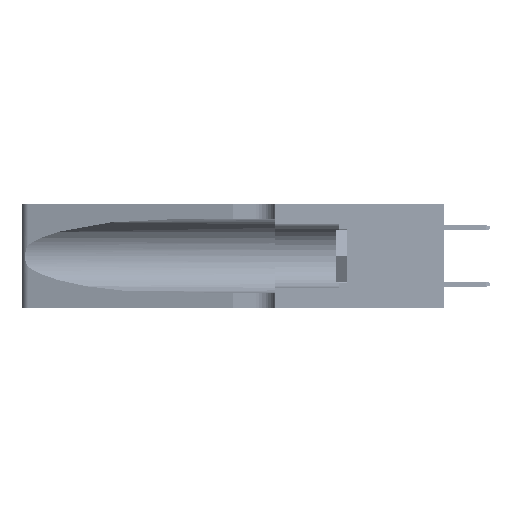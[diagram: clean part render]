
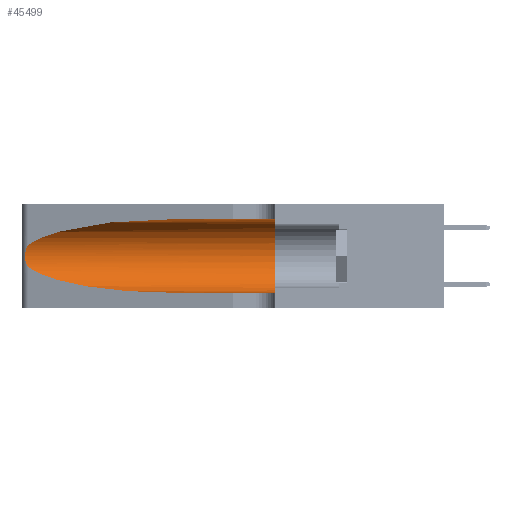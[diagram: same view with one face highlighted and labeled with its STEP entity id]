
A CAD part, left-side view. The second image highlights one B-rep face of the part: STEP entity #45499.
In plain terms, the highlighted cylindrical face has radius 3.308 mm (diameter 6.617 mm), a partial arc.
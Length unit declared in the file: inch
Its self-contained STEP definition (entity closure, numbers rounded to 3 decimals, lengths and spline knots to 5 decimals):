
#2262 = CARTESIAN_POINT ( 'NONE',  ( 0.26018, 1.23835, 0.19895 ) ) ;
#3183 =( BOUNDED_CURVE ( )  B_SPLINE_CURVE ( 3, ( #20846, #33221, #45657, #21023 ),
 .UNSPECIFIED., .F., .T. ) 
 B_SPLINE_CURVE_WITH_KNOTS ( ( 4, 4 ),
 ( 3.44316, 4.71239 ),
 .UNSPECIFIED. ) 
 CURVE ( )  GEOMETRIC_REPRESENTATION_ITEM ( )  RATIONAL_B_SPLINE_CURVE ( ( 1., 0.87, 0.87, 1. ) ) 
 REPRESENTATION_ITEM ( '' )  );
#4073 = DIRECTION ( 'NONE',  ( 0., 1., 0. ) ) ;
#5141 = VERTEX_POINT ( 'NONE', #37150 ) ;
#6443 = CARTESIAN_POINT ( 'NONE',  ( 0.26075, 1.23896, 0.178 ) ) ;
#7772 = ORIENTED_EDGE ( 'NONE', *, *, #43254, .T. ) ;
#9299 = CARTESIAN_POINT ( 'NONE',  ( 0.25487, 1.22718, 0.22369 ) ) ;
#9492 = CARTESIAN_POINT ( 'NONE',  ( 0.18966, 0.96281, 0.31525 ) ) ;
#10588 = CARTESIAN_POINT ( 'NONE',  ( 0.1305, 1.61858, 0.05475 ) ) ;
#10632 = CARTESIAN_POINT ( 'NONE',  ( 0.25856, 1.23593, 0.16098 ) ) ;
#12573 = EDGE_CURVE ( 'NONE', #46532, #25900, #16031, .T. ) ;
#13188 = FACE_OUTER_BOUND ( 'NONE', #14449, .T. ) ;
#13299 = CIRCLE ( 'NONE', #32196, 0.13025 ) ;
#13837 = CARTESIAN_POINT ( 'NONE',  ( 0.25487, 1.22718, 0.22369 ) ) ;
#14449 = EDGE_LOOP ( 'NONE', ( #7772, #16851, #31658, #46491, #23993, #29139 ) ) ;
#14777 = CARTESIAN_POINT ( 'NONE',  ( 0.25639, 1.23186, 0.15144 ) ) ;
#16031 = B_SPLINE_CURVE_WITH_KNOTS ( 'NONE', 3,
 ( #22903, #47535, #43394, #51656, #27020, #2262, #31151, #6443, #35260, #10632, #39422, #14777, #43569, #18944 ),
 .UNSPECIFIED., .F., .F.,
 ( 4, 2, 2, 2, 2, 2, 4 ),
 ( 0., 0.00027, 0.00053, 0.00107, 0.0016, 0.00187, 0.00214 ),
 .UNSPECIFIED. ) ;
#16258 = CARTESIAN_POINT ( 'NONE',  ( 0.1305, 0.72297, 0.31525 ) ) ;
#16335 = EDGE_CURVE ( 'NONE', #18346, #37292, #13299, .T. ) ;
#16851 = ORIENTED_EDGE ( 'NONE', *, *, #12573, .T. ) ;
#18346 = VERTEX_POINT ( 'NONE', #20769 ) ;
#18944 = CARTESIAN_POINT ( 'NONE',  ( 0.25487, 1.22718, 0.14631 ) ) ;
#20769 = CARTESIAN_POINT ( 'NONE',  ( 0.1305, 0.35, 0.31525 ) ) ;
#20846 = CARTESIAN_POINT ( 'NONE',  ( 0.25487, 1.22718, 0.14631 ) ) ;
#21023 = CARTESIAN_POINT ( 'NONE',  ( 0.1305, 0.72297, 0.05475 ) ) ;
#22903 = CARTESIAN_POINT ( 'NONE',  ( 0.25487, 1.22718, 0.22369 ) ) ;
#22929 = CARTESIAN_POINT ( 'NONE',  ( 0.1305, 1.61858, 0.31525 ) ) ;
#23993 = ORIENTED_EDGE ( 'NONE', *, *, #16335, .F. ) ;
#24260 = CARTESIAN_POINT ( 'NONE',  ( 0.25487, 1.22718, 0.14631 ) ) ;
#25882 = VECTOR ( 'NONE', #35219, 39.37008 ) ;
#25900 = VERTEX_POINT ( 'NONE', #24260 ) ;
#27020 = CARTESIAN_POINT ( 'NONE',  ( 0.25854, 1.2359, 0.20912 ) ) ;
#27040 = CARTESIAN_POINT ( 'NONE',  ( 0.1305, 1.61858, 0.185 ) ) ;
#28819 = CARTESIAN_POINT ( 'NONE',  ( 0.1305, 0.35, 0.185 ) ) ;
#29139 = ORIENTED_EDGE ( 'NONE', *, *, #37641, .F. ) ;
#29776 = VERTEX_POINT ( 'NONE', #16258 ) ;
#31151 = CARTESIAN_POINT ( 'NONE',  ( 0.26075, 1.23896, 0.19203 ) ) ;
#31658 = ORIENTED_EDGE ( 'NONE', *, *, #33226, .T. ) ;
#32196 = AXIS2_PLACEMENT_3D ( 'NONE', #28819, #4073, #32950 ) ;
#32897 = EDGE_CURVE ( 'NONE', #5141, #37292, #39372, .T. ) ;
#32950 = DIRECTION ( 'NONE',  ( 0., 0., 1. ) ) ;
#33221 = CARTESIAN_POINT ( 'NONE',  ( 0.2373, 1.15595, 0.08982 ) ) ;
#33226 = EDGE_CURVE ( 'NONE', #25900, #5141, #3183, .T. ) ;
#33771 = CYLINDRICAL_SURFACE ( 'NONE', #36055, 0.13025 ) ;
#34322 = CARTESIAN_POINT ( 'NONE',  ( 0.1305, 0.72297, 0.31525 ) ) ;
#35219 = DIRECTION ( 'NONE',  ( 0., -1., 0. ) ) ;
#35260 = CARTESIAN_POINT ( 'NONE',  ( 0.26017, 1.23833, 0.17102 ) ) ;
#35282 = DIRECTION ( 'NONE',  ( 0., -1., 0. ) ) ;
#35836 =( BOUNDED_CURVE ( )  B_SPLINE_CURVE ( 3, ( #34322, #9492, #38473, #13837 ),
 .UNSPECIFIED., .F., .F. ) 
 B_SPLINE_CURVE_WITH_KNOTS ( ( 4, 4 ),
 ( 1.5708, 2.84003 ),
 .UNSPECIFIED. ) 
 CURVE ( )  GEOMETRIC_REPRESENTATION_ITEM ( )  RATIONAL_B_SPLINE_CURVE ( ( 1., 0.87, 0.87, 1. ) ) 
 REPRESENTATION_ITEM ( '' )  );
#36055 = AXIS2_PLACEMENT_3D ( 'NONE', #27040, #35282, #47553 ) ;
#37150 = CARTESIAN_POINT ( 'NONE',  ( 0.1305, 0.72297, 0.05475 ) ) ;
#37292 = VERTEX_POINT ( 'NONE', #41225 ) ;
#37641 = EDGE_CURVE ( 'NONE', #29776, #18346, #51896, .T. ) ;
#38473 = CARTESIAN_POINT ( 'NONE',  ( 0.2373, 1.15595, 0.28018 ) ) ;
#39372 = LINE ( 'NONE', #10588, #25882 ) ;
#39422 = CARTESIAN_POINT ( 'NONE',  ( 0.25789, 1.23486, 0.15765 ) ) ;
#40940 = VECTOR ( 'NONE', #43593, 39.37008 ) ;
#41225 = CARTESIAN_POINT ( 'NONE',  ( 0.1305, 0.35, 0.05475 ) ) ;
#43254 = EDGE_CURVE ( 'NONE', #29776, #46532, #35836, .T. ) ;
#43394 = CARTESIAN_POINT ( 'NONE',  ( 0.25639, 1.23184, 0.21858 ) ) ;
#43569 = CARTESIAN_POINT ( 'NONE',  ( 0.25555, 1.22993, 0.14849 ) ) ;
#43593 = DIRECTION ( 'NONE',  ( 0., -1., 0. ) ) ;
#45499 = ADVANCED_FACE ( 'NONE', ( #13188 ), #33771, .F. ) ;
#45657 = CARTESIAN_POINT ( 'NONE',  ( 0.18966, 0.96281, 0.05475 ) ) ;
#46491 = ORIENTED_EDGE ( 'NONE', *, *, #32897, .T. ) ;
#46532 = VERTEX_POINT ( 'NONE', #9299 ) ;
#47535 = CARTESIAN_POINT ( 'NONE',  ( 0.25555, 1.22994, 0.2215 ) ) ;
#47553 = DIRECTION ( 'NONE',  ( 0., 0., -1. ) ) ;
#51656 = CARTESIAN_POINT ( 'NONE',  ( 0.25787, 1.23484, 0.2124 ) ) ;
#51896 = LINE ( 'NONE', #22929, #40940 ) ;
